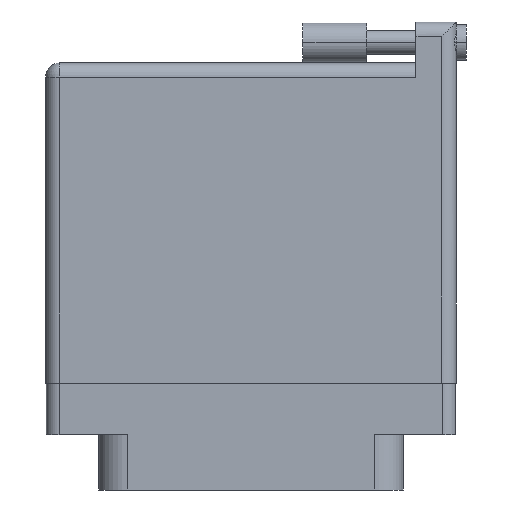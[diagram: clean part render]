
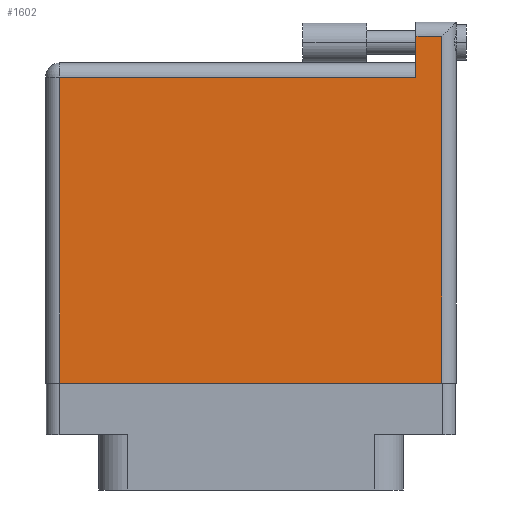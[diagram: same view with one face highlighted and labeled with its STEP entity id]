
A CAD part, front view. The second image highlights one B-rep face of the part: STEP entity #1602.
In plain terms, the highlighted face is planar.
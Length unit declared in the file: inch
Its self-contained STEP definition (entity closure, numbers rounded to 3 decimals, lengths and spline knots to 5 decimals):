
#304 = PLANE ( 'NONE',  #2446 ) ;
#1602 = ADVANCED_FACE ( 'NONE', ( #5810 ), #304, .F. ) ;
#1712 = LINE ( 'NONE', #8126, #2508 ) ;
#1733 = CARTESIAN_POINT ( 'NONE',  ( 0.807, 1.596, 0.4495 ) ) ;
#2083 = CARTESIAN_POINT ( 'NONE',  ( -0.934, 1.396, 0.4495 ) ) ;
#2446 = AXIS2_PLACEMENT_3D ( 'NONE', #17273, #2899, #17497 ) ;
#2508 = VECTOR ( 'NONE', #27930, 39.37008 ) ;
#2801 = CARTESIAN_POINT ( 'NONE',  ( 0.934, 1.666, 0.4495 ) ) ;
#2899 = DIRECTION ( 'NONE',  ( 0., 0., -1. ) ) ;
#3364 = LINE ( 'NONE', #2801, #12225 ) ;
#4028 = EDGE_CURVE ( 'NONE', #12607, #18779, #19818, .T. ) ;
#4344 = CARTESIAN_POINT ( 'NONE',  ( 0.807, 1.396, 0.4495 ) ) ;
#4569 = EDGE_CURVE ( 'NONE', #20610, #12607, #25206, .T. ) ;
#5810 = FACE_OUTER_BOUND ( 'NONE', #12705, .T. ) ;
#8126 = CARTESIAN_POINT ( 'NONE',  ( -1.004, -0.1, 0.4495 ) ) ;
#8301 = EDGE_CURVE ( 'NONE', #18779, #13823, #16200, .T. ) ;
#8960 = VERTEX_POINT ( 'NONE', #22108 ) ;
#9125 = CARTESIAN_POINT ( 'NONE',  ( 0.807, 1.666, 0.4495 ) ) ;
#9194 = CARTESIAN_POINT ( 'NONE',  ( -1.004, 1.396, 0.4495 ) ) ;
#9691 = VECTOR ( 'NONE', #30837, 39.37008 ) ;
#12225 = VECTOR ( 'NONE', #12280, 39.37008 ) ;
#12280 = DIRECTION ( 'NONE',  ( 0., 1., 0. ) ) ;
#12607 = VERTEX_POINT ( 'NONE', #1733 ) ;
#12705 = EDGE_LOOP ( 'NONE', ( #21657, #25388, #23646, #24807, #17377, #27445 ) ) ;
#13357 = VECTOR ( 'NONE', #28560, 39.37008 ) ;
#13823 = VERTEX_POINT ( 'NONE', #2083 ) ;
#14022 = VECTOR ( 'NONE', #16784, 39.37008 ) ;
#15573 = VECTOR ( 'NONE', #19332, 39.37008 ) ;
#16200 = LINE ( 'NONE', #9194, #9691 ) ;
#16679 = CARTESIAN_POINT ( 'NONE',  ( -1.004, 1.596, 0.4495 ) ) ;
#16784 = DIRECTION ( 'NONE',  ( -1., 0., 0. ) ) ;
#17273 = CARTESIAN_POINT ( 'NONE',  ( -1.004, 1.466, 0.4495 ) ) ;
#17377 = ORIENTED_EDGE ( 'NONE', *, *, #8301, .T. ) ;
#17497 = DIRECTION ( 'NONE',  ( -1., 0., 0. ) ) ;
#18421 = CARTESIAN_POINT ( 'NONE',  ( -0.934, -0.1, 0.4495 ) ) ;
#18779 = VERTEX_POINT ( 'NONE', #4344 ) ;
#19332 = DIRECTION ( 'NONE',  ( 0., -1., 0. ) ) ;
#19392 = CARTESIAN_POINT ( 'NONE',  ( 0.934, 1.596, 0.4495 ) ) ;
#19818 = LINE ( 'NONE', #9125, #15573 ) ;
#20610 = VERTEX_POINT ( 'NONE', #19392 ) ;
#21657 = ORIENTED_EDGE ( 'NONE', *, *, #24818, .T. ) ;
#21813 = CARTESIAN_POINT ( 'NONE',  ( 0.934, -0.1, 0.4495 ) ) ;
#22108 = CARTESIAN_POINT ( 'NONE',  ( -0.934, -0.1, 0.4495 ) ) ;
#22244 = LINE ( 'NONE', #18421, #13357 ) ;
#22790 = EDGE_CURVE ( 'NONE', #13823, #8960, #22244, .T. ) ;
#23646 = ORIENTED_EDGE ( 'NONE', *, *, #4569, .T. ) ;
#23967 = VERTEX_POINT ( 'NONE', #21813 ) ;
#24807 = ORIENTED_EDGE ( 'NONE', *, *, #4028, .T. ) ;
#24818 = EDGE_CURVE ( 'NONE', #8960, #23967, #1712, .T. ) ;
#25206 = LINE ( 'NONE', #16679, #14022 ) ;
#25388 = ORIENTED_EDGE ( 'NONE', *, *, #31986, .T. ) ;
#27445 = ORIENTED_EDGE ( 'NONE', *, *, #22790, .T. ) ;
#27930 = DIRECTION ( 'NONE',  ( 1., 0., 0. ) ) ;
#28560 = DIRECTION ( 'NONE',  ( 0., -1., 0. ) ) ;
#30837 = DIRECTION ( 'NONE',  ( -1., 0., 0. ) ) ;
#31986 = EDGE_CURVE ( 'NONE', #23967, #20610, #3364, .T. ) ;
